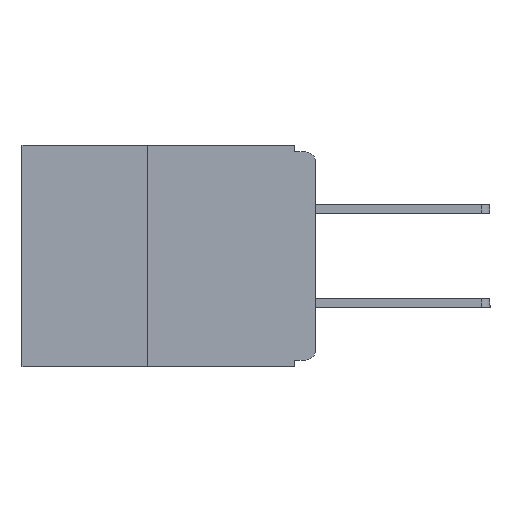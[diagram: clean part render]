
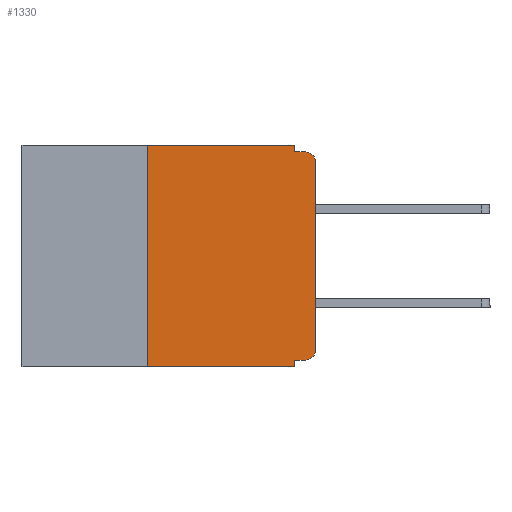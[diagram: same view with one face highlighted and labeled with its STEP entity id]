
A CAD part, left-side view. The second image highlights one B-rep face of the part: STEP entity #1330.
In plain terms, the highlighted planar face has unit normal (-1, 0, 0).
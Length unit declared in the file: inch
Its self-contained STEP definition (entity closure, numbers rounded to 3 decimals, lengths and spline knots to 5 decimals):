
#435 = DIRECTION ( 'NONE',  ( 0., 0., 1. ) ) ;
#505 = EDGE_CURVE ( 'NONE', #15804, #4234, #6944, .T. ) ;
#594 = CARTESIAN_POINT ( 'NONE',  ( 0., 0., -0.025 ) ) ;
#718 = VERTEX_POINT ( 'NONE', #12488 ) ;
#905 = CARTESIAN_POINT ( 'NONE',  ( 0., 0., -0.305 ) ) ;
#1088 = CARTESIAN_POINT ( 'NONE',  ( 0., 0.437, -0.33 ) ) ;
#1143 = VERTEX_POINT ( 'NONE', #9882 ) ;
#1330 = ADVANCED_FACE ( 'NONE', ( #15637 ), #9735, .F. ) ;
#2304 = VECTOR ( 'NONE', #12566, 39.37008 ) ;
#2599 = AXIS2_PLACEMENT_3D ( 'NONE', #14695, #6691, #15953 ) ;
#2713 = AXIS2_PLACEMENT_3D ( 'NONE', #11498, #11462, #11439 ) ;
#2795 = CARTESIAN_POINT ( 'NONE',  ( 0., 0.437, 0. ) ) ;
#3141 = DIRECTION ( 'NONE',  ( 0., -1., 0. ) ) ;
#3900 = VERTEX_POINT ( 'NONE', #8468 ) ;
#3979 = CIRCLE ( 'NONE', #2599, 0.015 ) ;
#3991 = VECTOR ( 'NONE', #3141, 39.37008 ) ;
#4234 = VERTEX_POINT ( 'NONE', #594 ) ;
#4729 = ORIENTED_EDGE ( 'NONE', *, *, #505, .T. ) ;
#4816 = EDGE_CURVE ( 'NONE', #8073, #15804, #17216, .T. ) ;
#4863 = LINE ( 'NONE', #7211, #11727 ) ;
#5218 = ORIENTED_EDGE ( 'NONE', *, *, #7590, .T. ) ;
#5764 = VECTOR ( 'NONE', #17316, 39.37008 ) ;
#5798 = LINE ( 'NONE', #12363, #15974 ) ;
#5800 = ORIENTED_EDGE ( 'NONE', *, *, #13898, .F. ) ;
#5849 = ORIENTED_EDGE ( 'NONE', *, *, #14829, .F. ) ;
#6398 = EDGE_CURVE ( 'NONE', #1143, #718, #10964, .T. ) ;
#6462 = DIRECTION ( 'NONE',  ( 0., 0., -1. ) ) ;
#6691 = DIRECTION ( 'NONE',  ( -1., 0., 0. ) ) ;
#6733 = ORIENTED_EDGE ( 'NONE', *, *, #6398, .F. ) ;
#6944 = LINE ( 'NONE', #9251, #17026 ) ;
#7211 = CARTESIAN_POINT ( 'NONE',  ( 0., 0.25, -0.33 ) ) ;
#7288 = ORIENTED_EDGE ( 'NONE', *, *, #13992, .F. ) ;
#7326 = ORIENTED_EDGE ( 'NONE', *, *, #13130, .T. ) ;
#7452 = ORIENTED_EDGE ( 'NONE', *, *, #12273, .F. ) ;
#7471 = CARTESIAN_POINT ( 'NONE',  ( 0., 0.25, -0.33 ) ) ;
#7487 = ORIENTED_EDGE ( 'NONE', *, *, #9453, .F. ) ;
#7590 = EDGE_CURVE ( 'NONE', #4234, #13753, #3979, .T. ) ;
#7887 = CARTESIAN_POINT ( 'NONE',  ( 0., 0.031, -0.33 ) ) ;
#8073 = VERTEX_POINT ( 'NONE', #9147 ) ;
#8204 = CARTESIAN_POINT ( 'NONE',  ( 0., 0.031, -0.32 ) ) ;
#8331 = CARTESIAN_POINT ( 'NONE',  ( 0., 0.437, 0. ) ) ;
#8468 = CARTESIAN_POINT ( 'NONE',  ( 0., 0.031, -0.01 ) ) ;
#8944 = VERTEX_POINT ( 'NONE', #8204 ) ;
#8961 = ORIENTED_EDGE ( 'NONE', *, *, #4816, .T. ) ;
#9147 = CARTESIAN_POINT ( 'NONE',  ( 0., 0.015, -0.32 ) ) ;
#9251 = CARTESIAN_POINT ( 'NONE',  ( 0., 0., 0. ) ) ;
#9453 = EDGE_CURVE ( 'NONE', #8073, #8944, #14344, .T. ) ;
#9705 = EDGE_LOOP ( 'NONE', ( #4729, #5218, #5800, #5849, #6733, #7288, #7326, #7452, #7487, #8961 ) ) ;
#9735 = PLANE ( 'NONE',  #12477 ) ;
#9882 = CARTESIAN_POINT ( 'NONE',  ( 0., 0.25, 0. ) ) ;
#10342 = CARTESIAN_POINT ( 'NONE',  ( 0., 0., -0.32 ) ) ;
#10621 = CARTESIAN_POINT ( 'NONE',  ( 0., 0.031, 0. ) ) ;
#10886 = VECTOR ( 'NONE', #11687, 39.37008 ) ;
#10911 = VERTEX_POINT ( 'NONE', #7887 ) ;
#10938 = CARTESIAN_POINT ( 'NONE',  ( 0., 0.015, -0.01 ) ) ;
#10964 = LINE ( 'NONE', #2795, #3991 ) ;
#11439 = DIRECTION ( 'NONE',  ( 0., 0., -1. ) ) ;
#11462 = DIRECTION ( 'NONE',  ( -1., 0., 0. ) ) ;
#11498 = CARTESIAN_POINT ( 'NONE',  ( 0., 0.015, -0.305 ) ) ;
#11687 = DIRECTION ( 'NONE',  ( 0., 1., 0. ) ) ;
#11727 = VECTOR ( 'NONE', #12734, 39.37008 ) ;
#12273 = EDGE_CURVE ( 'NONE', #8944, #10911, #5798, .T. ) ;
#12363 = CARTESIAN_POINT ( 'NONE',  ( 0., 0.031, -0.33 ) ) ;
#12477 = AXIS2_PLACEMENT_3D ( 'NONE', #8331, #14588, #16244 ) ;
#12488 = CARTESIAN_POINT ( 'NONE',  ( 0., 0.031, 0. ) ) ;
#12566 = DIRECTION ( 'NONE',  ( 0., -1., 0. ) ) ;
#12734 = DIRECTION ( 'NONE',  ( 0., 0., 1. ) ) ;
#13130 = EDGE_CURVE ( 'NONE', #16174, #10911, #16342, .T. ) ;
#13753 = VERTEX_POINT ( 'NONE', #10938 ) ;
#13898 = EDGE_CURVE ( 'NONE', #3900, #13753, #16688, .T. ) ;
#13932 = LINE ( 'NONE', #10621, #16843 ) ;
#13992 = EDGE_CURVE ( 'NONE', #16174, #1143, #4863, .T. ) ;
#14344 = LINE ( 'NONE', #10342, #10886 ) ;
#14588 = DIRECTION ( 'NONE',  ( 1., 0., 0. ) ) ;
#14695 = CARTESIAN_POINT ( 'NONE',  ( 0., 0.015, -0.025 ) ) ;
#14829 = EDGE_CURVE ( 'NONE', #718, #3900, #13932, .T. ) ;
#15637 = FACE_OUTER_BOUND ( 'NONE', #9705, .T. ) ;
#15804 = VERTEX_POINT ( 'NONE', #905 ) ;
#15953 = DIRECTION ( 'NONE',  ( 0., 0., -1. ) ) ;
#15974 = VECTOR ( 'NONE', #16167, 39.37008 ) ;
#16167 = DIRECTION ( 'NONE',  ( 0., 0., -1. ) ) ;
#16174 = VERTEX_POINT ( 'NONE', #7471 ) ;
#16244 = DIRECTION ( 'NONE',  ( 0., 0., -1. ) ) ;
#16330 = CARTESIAN_POINT ( 'NONE',  ( 0., 0., -0.01 ) ) ;
#16342 = LINE ( 'NONE', #1088, #5764 ) ;
#16688 = LINE ( 'NONE', #16330, #2304 ) ;
#16843 = VECTOR ( 'NONE', #6462, 39.37008 ) ;
#17026 = VECTOR ( 'NONE', #435, 39.37008 ) ;
#17216 = CIRCLE ( 'NONE', #2713, 0.015 ) ;
#17316 = DIRECTION ( 'NONE',  ( 0., -1., 0. ) ) ;
